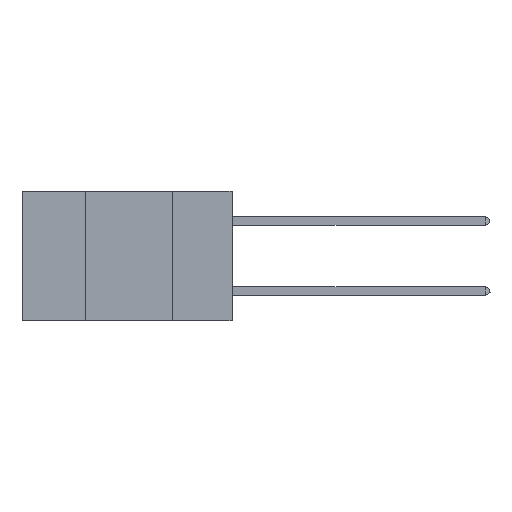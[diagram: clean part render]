
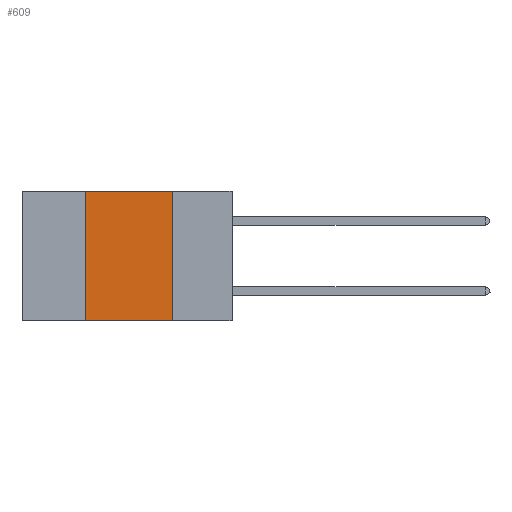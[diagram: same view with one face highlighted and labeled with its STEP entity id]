
A CAD part, left-side view. The second image highlights one B-rep face of the part: STEP entity #609.
In plain terms, the highlighted planar face has unit normal (-1, 0, 0).
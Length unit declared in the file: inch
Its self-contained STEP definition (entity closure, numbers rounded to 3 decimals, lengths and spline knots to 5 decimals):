
#15 = ORIENTED_EDGE ( 'NONE', *, *, #11174, .T. ) ;
#299 = CARTESIAN_POINT ( 'NONE',  ( 0., 0.6, 0. ) ) ;
#337 = VERTEX_POINT ( 'NONE', #11182 ) ;
#536 = CARTESIAN_POINT ( 'NONE',  ( 0., 0.42, 0. ) ) ;
#609 = ADVANCED_FACE ( 'NONE', ( #1368 ), #9444, .F. ) ;
#1021 = DIRECTION ( 'NONE',  ( 0., -1., 0. ) ) ;
#1098 = LINE ( 'NONE', #1162, #3845 ) ;
#1162 = CARTESIAN_POINT ( 'NONE',  ( 0., 0.6, 0. ) ) ;
#1163 = ORIENTED_EDGE ( 'NONE', *, *, #2047, .F. ) ;
#1346 = LINE ( 'NONE', #12426, #5115 ) ;
#1368 = FACE_OUTER_BOUND ( 'NONE', #2541, .T. ) ;
#1376 = EDGE_CURVE ( 'NONE', #7366, #3311, #1098, .T. ) ;
#2047 = EDGE_CURVE ( 'NONE', #3311, #337, #6880, .T. ) ;
#2316 = CARTESIAN_POINT ( 'NONE',  ( 0., 0.42, 0. ) ) ;
#2541 = EDGE_LOOP ( 'NONE', ( #1163, #3188, #10262, #15 ) ) ;
#2581 = VECTOR ( 'NONE', #10679, 39.37008 ) ;
#3188 = ORIENTED_EDGE ( 'NONE', *, *, #1376, .F. ) ;
#3283 = EDGE_CURVE ( 'NONE', #3936, #7366, #3603, .T. ) ;
#3311 = VERTEX_POINT ( 'NONE', #7546 ) ;
#3603 = LINE ( 'NONE', #536, #2581 ) ;
#3845 = VECTOR ( 'NONE', #1021, 39.37008 ) ;
#3936 = VERTEX_POINT ( 'NONE', #8798 ) ;
#4070 = VECTOR ( 'NONE', #11873, 39.37008 ) ;
#4365 = DIRECTION ( 'NONE',  ( 1., 0., 0. ) ) ;
#5115 = VECTOR ( 'NONE', #5218, 39.37008 ) ;
#5218 = DIRECTION ( 'NONE',  ( 0., -1., 0. ) ) ;
#6678 = CARTESIAN_POINT ( 'NONE',  ( 0., 0.17, 0. ) ) ;
#6880 = LINE ( 'NONE', #6678, #4070 ) ;
#7366 = VERTEX_POINT ( 'NONE', #2316 ) ;
#7546 = CARTESIAN_POINT ( 'NONE',  ( 0., 0.17, 0. ) ) ;
#8429 = DIRECTION ( 'NONE',  ( 0., 0., -1. ) ) ;
#8798 = CARTESIAN_POINT ( 'NONE',  ( 0., 0.42, -0.37 ) ) ;
#9444 = PLANE ( 'NONE',  #11265 ) ;
#10262 = ORIENTED_EDGE ( 'NONE', *, *, #3283, .F. ) ;
#10679 = DIRECTION ( 'NONE',  ( 0., 0., 1. ) ) ;
#11174 = EDGE_CURVE ( 'NONE', #3936, #337, #1346, .T. ) ;
#11182 = CARTESIAN_POINT ( 'NONE',  ( 0., 0.17, -0.37 ) ) ;
#11265 = AXIS2_PLACEMENT_3D ( 'NONE', #299, #4365, #8429 ) ;
#11873 = DIRECTION ( 'NONE',  ( 0., 0., -1. ) ) ;
#12426 = CARTESIAN_POINT ( 'NONE',  ( 0., 0.6, -0.37 ) ) ;
